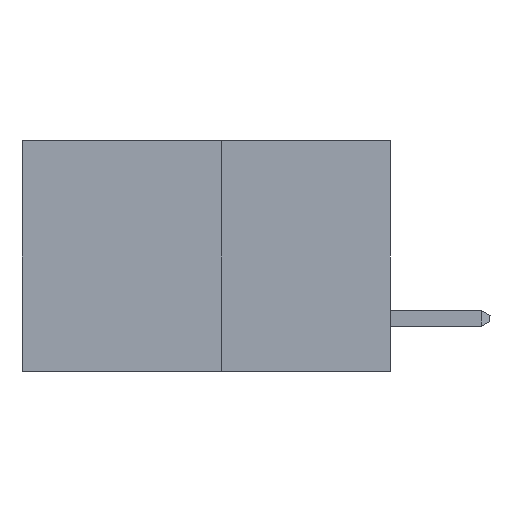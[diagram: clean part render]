
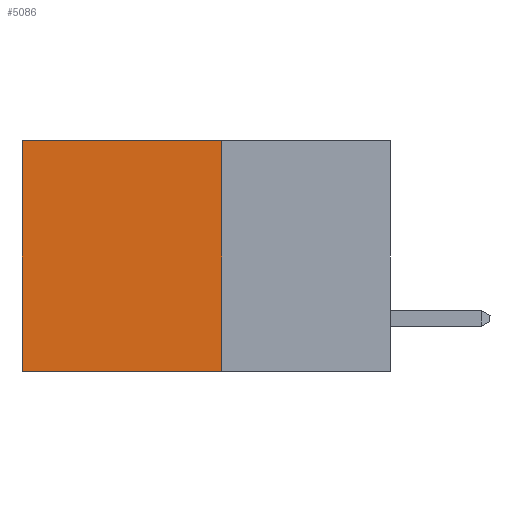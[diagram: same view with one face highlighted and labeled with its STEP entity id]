
A CAD part, left-side view. The second image highlights one B-rep face of the part: STEP entity #5086.
In plain terms, the highlighted planar face has unit normal (-1, 0, 0).
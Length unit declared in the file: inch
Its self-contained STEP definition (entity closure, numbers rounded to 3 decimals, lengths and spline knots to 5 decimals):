
#476 = CARTESIAN_POINT ( 'NONE',  ( 0.277, 0.27, -0.37 ) ) ;
#480 = DIRECTION ( 'NONE',  ( 0., 0., -1. ) ) ;
#491 = DIRECTION ( 'NONE',  ( 0., 1., 0. ) ) ;
#521 = VERTEX_POINT ( 'NONE', #5721 ) ;
#1072 = EDGE_CURVE ( 'NONE', #7300, #6303, #3332, .T. ) ;
#1131 = VERTEX_POINT ( 'NONE', #1196 ) ;
#1196 = CARTESIAN_POINT ( 'NONE',  ( 0.277, 0.59, -0.37 ) ) ;
#1475 = VECTOR ( 'NONE', #6189, 39.37008 ) ;
#1925 = DIRECTION ( 'NONE',  ( 1., 0., 0. ) ) ;
#2179 = VECTOR ( 'NONE', #491, 39.37008 ) ;
#2276 = CARTESIAN_POINT ( 'NONE',  ( 0.277, 0.27, 0. ) ) ;
#2897 = DIRECTION ( 'NONE',  ( 0., 0., -1. ) ) ;
#3070 = CARTESIAN_POINT ( 'NONE',  ( 0.277, 0.27, -0.37 ) ) ;
#3113 = EDGE_CURVE ( 'NONE', #6303, #1131, #8624, .T. ) ;
#3164 = CARTESIAN_POINT ( 'NONE',  ( 0.277, 0.27, 0. ) ) ;
#3332 = LINE ( 'NONE', #2276, #1475 ) ;
#3388 = VECTOR ( 'NONE', #2897, 39.37008 ) ;
#3504 = EDGE_CURVE ( 'NONE', #521, #1131, #5786, .T. ) ;
#4296 = PLANE ( 'NONE',  #6508 ) ;
#4403 = CARTESIAN_POINT ( 'NONE',  ( 0.277, 0.27, -0.37 ) ) ;
#4597 = ORIENTED_EDGE ( 'NONE', *, *, #3113, .T. ) ;
#4786 = CARTESIAN_POINT ( 'NONE',  ( 0.277, 0.59, 0. ) ) ;
#4939 = ORIENTED_EDGE ( 'NONE', *, *, #3504, .F. ) ;
#5086 = ADVANCED_FACE ( 'NONE', ( #7268 ), #4296, .F. ) ;
#5219 = ORIENTED_EDGE ( 'NONE', *, *, #7073, .F. ) ;
#5721 = CARTESIAN_POINT ( 'NONE',  ( 0.277, 0.27, -0.37 ) ) ;
#5786 = LINE ( 'NONE', #476, #2179 ) ;
#6189 = DIRECTION ( 'NONE',  ( 0., 1., 0. ) ) ;
#6303 = VERTEX_POINT ( 'NONE', #4786 ) ;
#6322 = ORIENTED_EDGE ( 'NONE', *, *, #1072, .T. ) ;
#6508 = AXIS2_PLACEMENT_3D ( 'NONE', #3070, #1925, #480 ) ;
#6550 = VECTOR ( 'NONE', #8707, 39.37008 ) ;
#7073 = EDGE_CURVE ( 'NONE', #7300, #521, #8282, .T. ) ;
#7268 = FACE_OUTER_BOUND ( 'NONE', #8079, .T. ) ;
#7300 = VERTEX_POINT ( 'NONE', #3164 ) ;
#8079 = EDGE_LOOP ( 'NONE', ( #4597, #4939, #5219, #6322 ) ) ;
#8282 = LINE ( 'NONE', #4403, #6550 ) ;
#8459 = CARTESIAN_POINT ( 'NONE',  ( 0.277, 0.59, -0.37 ) ) ;
#8624 = LINE ( 'NONE', #8459, #3388 ) ;
#8707 = DIRECTION ( 'NONE',  ( 0., 0., -1. ) ) ;
